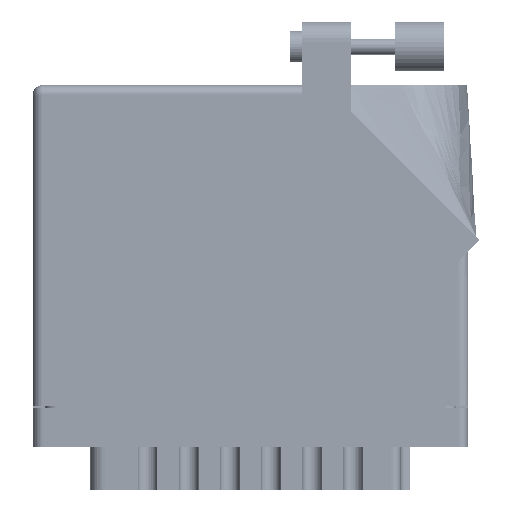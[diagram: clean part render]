
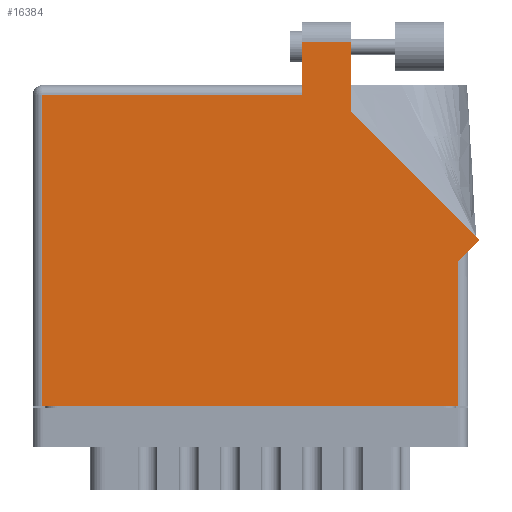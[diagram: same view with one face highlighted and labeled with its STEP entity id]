
A CAD part, front view. The second image highlights one B-rep face of the part: STEP entity #16384.
In plain terms, the highlighted face is planar.
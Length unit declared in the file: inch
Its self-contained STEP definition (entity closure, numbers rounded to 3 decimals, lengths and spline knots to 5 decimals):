
#416 = VERTEX_POINT ( 'NONE', #20910 ) ;
#2415 = DIRECTION ( 'NONE',  ( -0.707, 0.707, 0. ) ) ;
#3752 = EDGE_LOOP ( 'NONE', ( #61141, #73078, #74630, #39030, #47200, #47172, #42412, #84952, #84264 ) ) ;
#4552 = VECTOR ( 'NONE', #63792, 39.37008 ) ;
#5670 = CARTESIAN_POINT ( 'NONE',  ( 1.705, 2.03, 0. ) ) ;
#7097 = DIRECTION ( 'NONE',  ( -1., 0., 0. ) ) ;
#9079 = LINE ( 'NONE', #45249, #56335 ) ;
#11823 = VECTOR ( 'NONE', #7097, 39.37008 ) ;
#12289 = DIRECTION ( 'NONE',  ( 0., -1., 0. ) ) ;
#16384 = ADVANCED_FACE ( 'NONE', ( #66083 ), #52640, .F. ) ;
#16619 = EDGE_CURVE ( 'NONE', #63940, #38313, #85020, .T. ) ;
#17349 = EDGE_CURVE ( 'NONE', #64850, #63940, #86047, .T. ) ;
#20910 = CARTESIAN_POINT ( 'NONE',  ( 2.012, 2.305, 0. ) ) ;
#21631 = EDGE_CURVE ( 'NONE', #70453, #82302, #45031, .T. ) ;
#22795 = VECTOR ( 'NONE', #12289, 39.37008 ) ;
#23436 = VECTOR ( 'NONE', #39035, 39.37008 ) ;
#23669 = DIRECTION ( 'NONE',  ( -1., 0., 0. ) ) ;
#26005 = CARTESIAN_POINT ( 'NONE',  ( 2.012, 1.86442, 0. ) ) ;
#26966 = EDGE_CURVE ( 'NONE', #74338, #64850, #67370, .T. ) ;
#27471 = CARTESIAN_POINT ( 'NONE',  ( 2.693, 0.918, 0. ) ) ;
#27491 = CARTESIAN_POINT ( 'NONE',  ( 2.82571, 1.05071, 0. ) ) ;
#29536 = DIRECTION ( 'NONE',  ( 0., 1., 0. ) ) ;
#30703 = CARTESIAN_POINT ( 'NONE',  ( 2.693, 0., 0. ) ) ;
#31000 = LINE ( 'NONE', #44182, #11823 ) ;
#35054 = VECTOR ( 'NONE', #2415, 39.37008 ) ;
#37571 = CARTESIAN_POINT ( 'NONE',  ( 0., 2.03, 0. ) ) ;
#37974 = CARTESIAN_POINT ( 'NONE',  ( 0.062, 0., 0. ) ) ;
#38313 = VERTEX_POINT ( 'NONE', #27491 ) ;
#39030 = ORIENTED_EDGE ( 'NONE', *, *, #53800, .T. ) ;
#39035 = DIRECTION ( 'NONE',  ( 1., 0., 0. ) ) ;
#42412 = ORIENTED_EDGE ( 'NONE', *, *, #17349, .T. ) ;
#44182 = CARTESIAN_POINT ( 'NONE',  ( 0., 1.968, 0. ) ) ;
#45031 = LINE ( 'NONE', #5670, #4552 ) ;
#45249 = CARTESIAN_POINT ( 'NONE',  ( 1.705, 2.305, 0. ) ) ;
#47172 = ORIENTED_EDGE ( 'NONE', *, *, #26966, .T. ) ;
#47200 = ORIENTED_EDGE ( 'NONE', *, *, #67424, .T. ) ;
#48053 = VECTOR ( 'NONE', #76735, 39.37008 ) ;
#50986 = LINE ( 'NONE', #83616, #22795 ) ;
#51087 = CARTESIAN_POINT ( 'NONE',  ( 2.012, 1.86442, 0. ) ) ;
#52143 = EDGE_CURVE ( 'NONE', #55912, #416, #87315, .T. ) ;
#52470 = DIRECTION ( 'NONE',  ( -1., 0., 0. ) ) ;
#52604 = CARTESIAN_POINT ( 'NONE',  ( 1.705, 1.968, 0. ) ) ;
#52640 = PLANE ( 'NONE',  #84174 ) ;
#53800 = EDGE_CURVE ( 'NONE', #82302, #76627, #31000, .T. ) ;
#55912 = VERTEX_POINT ( 'NONE', #26005 ) ;
#56335 = VECTOR ( 'NONE', #52470, 39.37008 ) ;
#58938 = DIRECTION ( 'NONE',  ( 0., 1., 0. ) ) ;
#61141 = ORIENTED_EDGE ( 'NONE', *, *, #52143, .T. ) ;
#63792 = DIRECTION ( 'NONE',  ( 0., -1., 0. ) ) ;
#63940 = VERTEX_POINT ( 'NONE', #27471 ) ;
#64850 = VERTEX_POINT ( 'NONE', #30703 ) ;
#66083 = FACE_OUTER_BOUND ( 'NONE', #3752, .T. ) ;
#67088 = CARTESIAN_POINT ( 'NONE',  ( 2.82571, 1.05071, 0. ) ) ;
#67370 = LINE ( 'NONE', #73871, #23436 ) ;
#67424 = EDGE_CURVE ( 'NONE', #76627, #74338, #50986, .T. ) ;
#70447 = CARTESIAN_POINT ( 'NONE',  ( 2.755, 0.98, 0. ) ) ;
#70453 = VERTEX_POINT ( 'NONE', #82953 ) ;
#71677 = EDGE_CURVE ( 'NONE', #38313, #55912, #75487, .T. ) ;
#73078 = ORIENTED_EDGE ( 'NONE', *, *, #92523, .T. ) ;
#73451 = CARTESIAN_POINT ( 'NONE',  ( 2.693, 0.98, 0. ) ) ;
#73871 = CARTESIAN_POINT ( 'NONE',  ( 0., 0., 0. ) ) ;
#74338 = VERTEX_POINT ( 'NONE', #37974 ) ;
#74630 = ORIENTED_EDGE ( 'NONE', *, *, #21631, .T. ) ;
#75487 = LINE ( 'NONE', #67088, #35054 ) ;
#76627 = VERTEX_POINT ( 'NONE', #91978 ) ;
#76735 = DIRECTION ( 'NONE',  ( 0.707, 0.707, 0. ) ) ;
#82302 = VERTEX_POINT ( 'NONE', #52604 ) ;
#82953 = CARTESIAN_POINT ( 'NONE',  ( 1.705, 2.305, 0. ) ) ;
#83616 = CARTESIAN_POINT ( 'NONE',  ( 0.062, 0., 0. ) ) ;
#84174 = AXIS2_PLACEMENT_3D ( 'NONE', #37571, #88027, #23669 ) ;
#84264 = ORIENTED_EDGE ( 'NONE', *, *, #71677, .T. ) ;
#84952 = ORIENTED_EDGE ( 'NONE', *, *, #16619, .T. ) ;
#85020 = LINE ( 'NONE', #70447, #48053 ) ;
#86047 = LINE ( 'NONE', #73451, #91655 ) ;
#86264 = VECTOR ( 'NONE', #58938, 39.37008 ) ;
#87315 = LINE ( 'NONE', #51087, #86264 ) ;
#88027 = DIRECTION ( 'NONE',  ( 0., 0., -1. ) ) ;
#91655 = VECTOR ( 'NONE', #29536, 39.37008 ) ;
#91978 = CARTESIAN_POINT ( 'NONE',  ( 0.062, 1.968, 0. ) ) ;
#92523 = EDGE_CURVE ( 'NONE', #416, #70453, #9079, .T. ) ;
